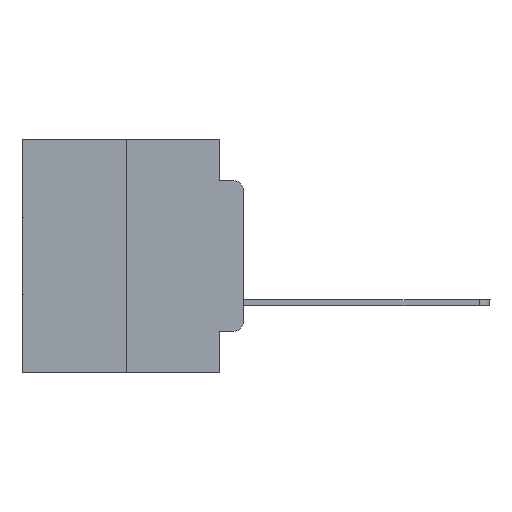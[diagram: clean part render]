
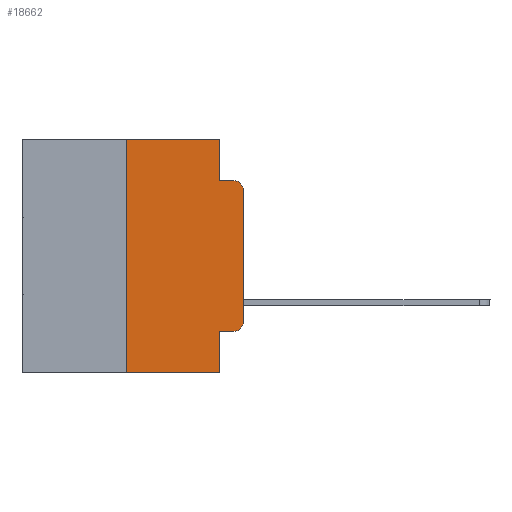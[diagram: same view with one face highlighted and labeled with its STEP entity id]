
A CAD part, left-side view. The second image highlights one B-rep face of the part: STEP entity #18662.
In plain terms, the highlighted planar face has unit normal (-1, 0, 0).
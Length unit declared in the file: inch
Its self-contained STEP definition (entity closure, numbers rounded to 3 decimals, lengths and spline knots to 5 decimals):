
#329 = PLANE ( 'NONE',  #9253 ) ;
#837 = LINE ( 'NONE', #13671, #14170 ) ;
#1322 = CARTESIAN_POINT ( 'NONE',  ( 0., 0., 0. ) ) ;
#2445 = EDGE_CURVE ( 'NONE', #17409, #16919, #17280, .T. ) ;
#2587 = CARTESIAN_POINT ( 'NONE',  ( 0., 0.051, 0. ) ) ;
#3127 = CARTESIAN_POINT ( 'NONE',  ( 0., 0.051, 0. ) ) ;
#4153 = EDGE_CURVE ( 'NONE', #15270, #15995, #837, .T. ) ;
#4536 = ORIENTED_EDGE ( 'NONE', *, *, #5910, .F. ) ;
#4573 = DIRECTION ( 'NONE',  ( 0., -1., 0. ) ) ;
#4684 = VERTEX_POINT ( 'NONE', #11865 ) ;
#4710 = LINE ( 'NONE', #21909, #21399 ) ;
#4768 = CARTESIAN_POINT ( 'NONE',  ( 0., 0.02, -0.0885 ) ) ;
#5100 = DIRECTION ( 'NONE',  ( 0., -1., 0. ) ) ;
#5782 = AXIS2_PLACEMENT_3D ( 'NONE', #15196, #19585, #11015 ) ;
#5910 = EDGE_CURVE ( 'NONE', #15270, #20396, #21753, .T. ) ;
#6074 = EDGE_CURVE ( 'NONE', #17103, #22351, #4710, .T. ) ;
#6622 = EDGE_CURVE ( 'NONE', #22351, #16919, #11681, .T. ) ;
#6712 = LINE ( 'NONE', #1322, #27086 ) ;
#6775 = CARTESIAN_POINT ( 'NONE',  ( 0., 0.25, -0.5 ) ) ;
#6900 = DIRECTION ( 'NONE',  ( 1., 0., 0. ) ) ;
#7227 = CARTESIAN_POINT ( 'NONE',  ( 0., 0.051, -0.0885 ) ) ;
#7384 = CARTESIAN_POINT ( 'NONE',  ( 0., 0., -0.1085 ) ) ;
#7721 = ORIENTED_EDGE ( 'NONE', *, *, #4153, .T. ) ;
#7819 = LINE ( 'NONE', #3127, #23175 ) ;
#7826 = DIRECTION ( 'NONE',  ( 0., 0., 1. ) ) ;
#8538 = ORIENTED_EDGE ( 'NONE', *, *, #16422, .T. ) ;
#8679 = ORIENTED_EDGE ( 'NONE', *, *, #6074, .F. ) ;
#9253 = AXIS2_PLACEMENT_3D ( 'NONE', #19703, #6900, #13626 ) ;
#9640 = CARTESIAN_POINT ( 'NONE',  ( 0., 0.02, -0.3915 ) ) ;
#9994 = VERTEX_POINT ( 'NONE', #23601 ) ;
#10477 = CARTESIAN_POINT ( 'NONE',  ( 0., 0.051, -0.4115 ) ) ;
#10689 = ORIENTED_EDGE ( 'NONE', *, *, #6622, .F. ) ;
#10724 = LINE ( 'NONE', #10477, #20051 ) ;
#10846 = ORIENTED_EDGE ( 'NONE', *, *, #20108, .T. ) ;
#11015 = DIRECTION ( 'NONE',  ( 0., 0., -1. ) ) ;
#11616 = CARTESIAN_POINT ( 'NONE',  ( 0., 0.051, -0.5 ) ) ;
#11681 = LINE ( 'NONE', #7227, #16365 ) ;
#11865 = CARTESIAN_POINT ( 'NONE',  ( 0., 0.02, -0.4115 ) ) ;
#12432 = FACE_OUTER_BOUND ( 'NONE', #24068, .T. ) ;
#12701 = CARTESIAN_POINT ( 'NONE',  ( 0., 0.051, -0.4115 ) ) ;
#12950 = EDGE_CURVE ( 'NONE', #27375, #15995, #7819, .T. ) ;
#13349 = AXIS2_PLACEMENT_3D ( 'NONE', #9640, #24932, #24560 ) ;
#13626 = DIRECTION ( 'NONE',  ( 0., 0., -1. ) ) ;
#13671 = CARTESIAN_POINT ( 'NONE',  ( 0., 0.473, -0.5 ) ) ;
#13780 = DIRECTION ( 'NONE',  ( 0., -1., 0. ) ) ;
#14170 = VECTOR ( 'NONE', #5100, 39.37008 ) ;
#14332 = ORIENTED_EDGE ( 'NONE', *, *, #2445, .T. ) ;
#14765 = DIRECTION ( 'NONE',  ( 0., -1., 0. ) ) ;
#15196 = CARTESIAN_POINT ( 'NONE',  ( 0., 0.02, -0.1085 ) ) ;
#15270 = VERTEX_POINT ( 'NONE', #6775 ) ;
#15536 = CARTESIAN_POINT ( 'NONE',  ( 0., 0.25, 0. ) ) ;
#15698 = DIRECTION ( 'NONE',  ( 0., 0., -1. ) ) ;
#15995 = VERTEX_POINT ( 'NONE', #11616 ) ;
#16365 = VECTOR ( 'NONE', #13780, 39.37008 ) ;
#16422 = EDGE_CURVE ( 'NONE', #4684, #9994, #27239, .T. ) ;
#16844 = LINE ( 'NONE', #17347, #23179 ) ;
#16919 = VERTEX_POINT ( 'NONE', #4768 ) ;
#17103 = VERTEX_POINT ( 'NONE', #2587 ) ;
#17280 = CIRCLE ( 'NONE', #5782, 0.02 ) ;
#17347 = CARTESIAN_POINT ( 'NONE',  ( 0., 0.473, 0. ) ) ;
#17409 = VERTEX_POINT ( 'NONE', #7384 ) ;
#18662 = ADVANCED_FACE ( 'NONE', ( #12432 ), #329, .F. ) ;
#18781 = DIRECTION ( 'NONE',  ( 0., 0., 1. ) ) ;
#19085 = VECTOR ( 'NONE', #18781, 39.37008 ) ;
#19585 = DIRECTION ( 'NONE',  ( -1., 0., 0. ) ) ;
#19703 = CARTESIAN_POINT ( 'NONE',  ( 0., 0.473, 0. ) ) ;
#20051 = VECTOR ( 'NONE', #14765, 39.37008 ) ;
#20108 = EDGE_CURVE ( 'NONE', #27375, #4684, #10724, .T. ) ;
#20231 = ORIENTED_EDGE ( 'NONE', *, *, #23308, .F. ) ;
#20396 = VERTEX_POINT ( 'NONE', #15536 ) ;
#21399 = VECTOR ( 'NONE', #23887, 39.37008 ) ;
#21753 = LINE ( 'NONE', #24928, #19085 ) ;
#21909 = CARTESIAN_POINT ( 'NONE',  ( 0., 0.051, 0. ) ) ;
#22016 = ORIENTED_EDGE ( 'NONE', *, *, #26110, .T. ) ;
#22351 = VERTEX_POINT ( 'NONE', #23567 ) ;
#23175 = VECTOR ( 'NONE', #15698, 39.37008 ) ;
#23179 = VECTOR ( 'NONE', #4573, 39.37008 ) ;
#23209 = ORIENTED_EDGE ( 'NONE', *, *, #12950, .F. ) ;
#23308 = EDGE_CURVE ( 'NONE', #20396, #17103, #16844, .T. ) ;
#23567 = CARTESIAN_POINT ( 'NONE',  ( 0., 0.051, -0.0885 ) ) ;
#23601 = CARTESIAN_POINT ( 'NONE',  ( 0., 0., -0.3915 ) ) ;
#23887 = DIRECTION ( 'NONE',  ( 0., 0., -1. ) ) ;
#24068 = EDGE_LOOP ( 'NONE', ( #22016, #14332, #10689, #8679, #20231, #4536, #7721, #23209, #10846, #8538 ) ) ;
#24560 = DIRECTION ( 'NONE',  ( 0., 0., -1. ) ) ;
#24928 = CARTESIAN_POINT ( 'NONE',  ( 0., 0.25, 0. ) ) ;
#24932 = DIRECTION ( 'NONE',  ( -1., 0., 0. ) ) ;
#26110 = EDGE_CURVE ( 'NONE', #9994, #17409, #6712, .T. ) ;
#27086 = VECTOR ( 'NONE', #7826, 39.37008 ) ;
#27239 = CIRCLE ( 'NONE', #13349, 0.02 ) ;
#27375 = VERTEX_POINT ( 'NONE', #12701 ) ;
